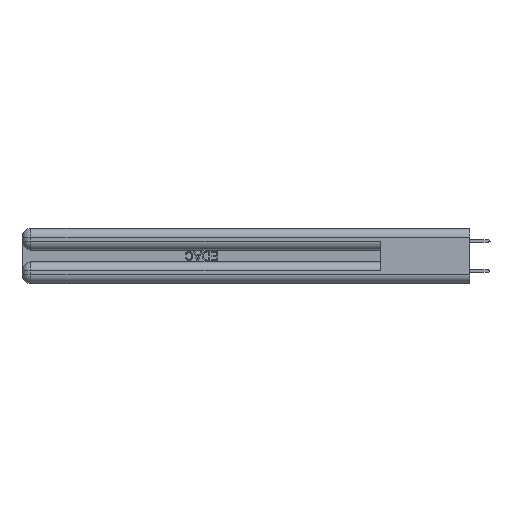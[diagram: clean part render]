
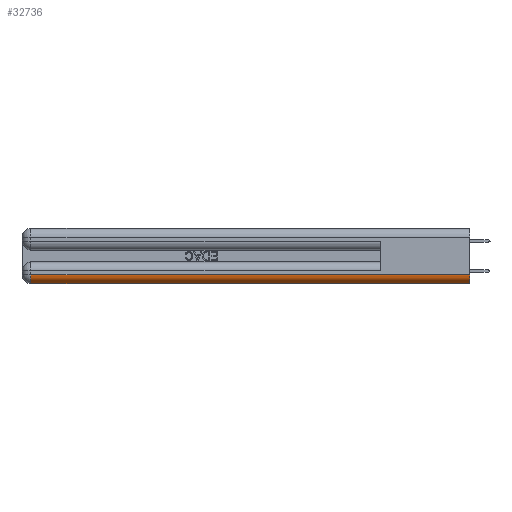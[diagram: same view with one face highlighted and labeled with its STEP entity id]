
A CAD part, left-side view. The second image highlights one B-rep face of the part: STEP entity #32736.
In plain terms, the highlighted cylindrical face has radius 1.524 mm (diameter 3.048 mm), a partial arc.
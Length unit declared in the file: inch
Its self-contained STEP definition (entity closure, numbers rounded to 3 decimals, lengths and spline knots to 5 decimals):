
#897 = DIRECTION ( 'NONE',  ( 0., 0., 1. ) ) ;
#2918 = VERTEX_POINT ( 'NONE', #3468 ) ;
#3468 = CARTESIAN_POINT ( 'NONE',  ( 0.06, 2.94, 0. ) ) ;
#3718 = AXIS2_PLACEMENT_3D ( 'NONE', #39289, #9714, #22834 ) ;
#4106 = DIRECTION ( 'NONE',  ( 0., 1., 0. ) ) ;
#4149 = DIRECTION ( 'NONE',  ( 0., -1., 0. ) ) ;
#4454 = VECTOR ( 'NONE', #4149, 39.37008 ) ;
#5156 = VERTEX_POINT ( 'NONE', #42653 ) ;
#5258 = VERTEX_POINT ( 'NONE', #42221 ) ;
#5260 = ORIENTED_EDGE ( 'NONE', *, *, #8374, .F. ) ;
#6553 = ORIENTED_EDGE ( 'NONE', *, *, #36528, .F. ) ;
#7359 = CARTESIAN_POINT ( 'NONE',  ( 0.06, 3., 0. ) ) ;
#7407 = CARTESIAN_POINT ( 'NONE',  ( 0., 0., 0.06 ) ) ;
#7996 = EDGE_CURVE ( 'NONE', #20613, #5156, #41033, .T. ) ;
#8374 = EDGE_CURVE ( 'NONE', #5258, #20613, #14490, .T. ) ;
#8533 = AXIS2_PLACEMENT_3D ( 'NONE', #13286, #23430, #897 ) ;
#9714 = DIRECTION ( 'NONE',  ( 0., -1., 0. ) ) ;
#10016 = CARTESIAN_POINT ( 'NONE',  ( 0., 0., 0.06 ) ) ;
#10340 = EDGE_CURVE ( 'NONE', #5156, #2918, #16438, .T. ) ;
#13286 = CARTESIAN_POINT ( 'NONE',  ( 0.06, 2.94, 0.06 ) ) ;
#13588 = ORIENTED_EDGE ( 'NONE', *, *, #10340, .F. ) ;
#14490 = LINE ( 'NONE', #7407, #4454 ) ;
#16209 = FACE_OUTER_BOUND ( 'NONE', #27674, .T. ) ;
#16438 = LINE ( 'NONE', #7359, #22863 ) ;
#19038 = CARTESIAN_POINT ( 'NONE',  ( 0.06, 0., 0.06 ) ) ;
#20613 = VERTEX_POINT ( 'NONE', #10016 ) ;
#22834 = DIRECTION ( 'NONE',  ( 0., 0., 1. ) ) ;
#22863 = VECTOR ( 'NONE', #4106, 39.37008 ) ;
#23430 = DIRECTION ( 'NONE',  ( 0., 1., 0. ) ) ;
#27205 = CIRCLE ( 'NONE', #8533, 0.06 ) ;
#27674 = EDGE_LOOP ( 'NONE', ( #33418, #5260, #6553, #13588 ) ) ;
#28363 = AXIS2_PLACEMENT_3D ( 'NONE', #19038, #29829, #29634 ) ;
#29634 = DIRECTION ( 'NONE',  ( 0., 0., 1. ) ) ;
#29829 = DIRECTION ( 'NONE',  ( 0., 1., 0. ) ) ;
#32736 = ADVANCED_FACE ( 'NONE', ( #16209 ), #39154, .T. ) ;
#33418 = ORIENTED_EDGE ( 'NONE', *, *, #7996, .F. ) ;
#36528 = EDGE_CURVE ( 'NONE', #2918, #5258, #27205, .T. ) ;
#39154 = CYLINDRICAL_SURFACE ( 'NONE', #28363, 0.06 ) ;
#39289 = CARTESIAN_POINT ( 'NONE',  ( 0.06, 0., 0.06 ) ) ;
#41033 = CIRCLE ( 'NONE', #3718, 0.06 ) ;
#42221 = CARTESIAN_POINT ( 'NONE',  ( 0., 2.94, 0.06 ) ) ;
#42653 = CARTESIAN_POINT ( 'NONE',  ( 0.06, 0., 0. ) ) ;
